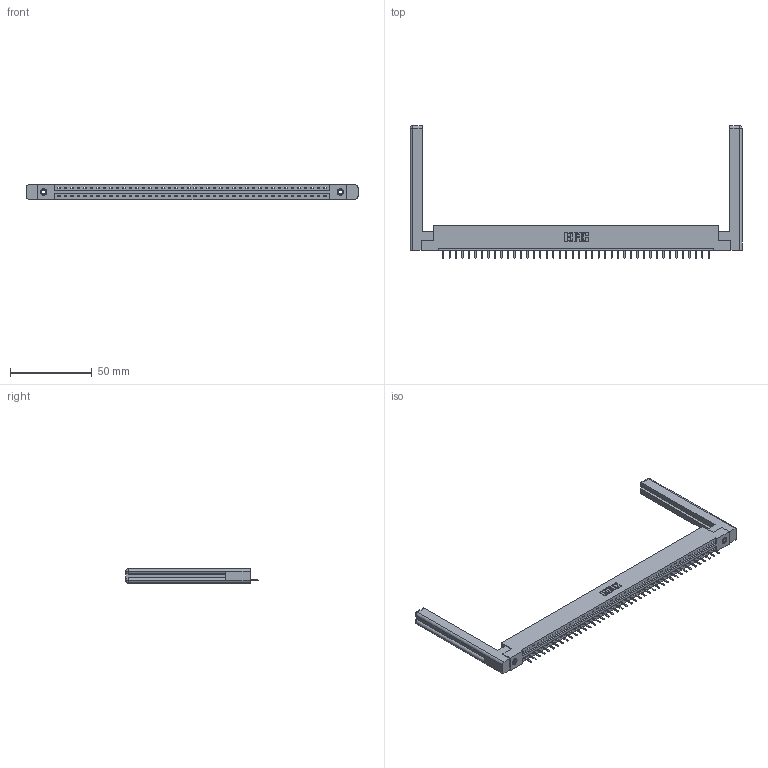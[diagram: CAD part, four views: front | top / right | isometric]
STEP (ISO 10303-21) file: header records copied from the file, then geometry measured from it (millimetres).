
FILE_DESCRIPTION (( 'STEP AP203' ), '1' );
FILE_NAME ('387-042-520-158.STEP', '2019-10-04T20:26:31', ( '' ), ( '' ), 'SwSTEP 2.0', 'SolidWorks 2016', '' );
FILE_SCHEMA (( 'CONFIG_CONTROL_DESIGN' ));
Length unit declared in the file: inch
Products named in the file (5): 345-292-001_345-293-120; 307-220-058; 345-250-001_345-250-001-102; 387-042-520-158; 337 Part_Flush Mounting Lugs - 0.156 Dia-TI
Assembly tree (47 placements, depth 2):
  387-042-520-158
    337 Part_Flush Mounting Lugs - 0.156 Dia-TI
    345-292-001_345-293-120  x42
    345-250-001_345-250-001-102  x2
    307-220-058  x2
Bounding box: 203.05 x 81.11 x 9.4 mm (x, y, z)
Volume: 28144.7 mm3; surface area: 26460.5 mm2
Topology: 47 solids, 47 shells, 3028 faces, 8897 edges, 5806 vertices
Faces by surface type: plane 2170, cylinder 834, cone 12, torus 12
Entity records: 33968 total; most frequent: CARTESIAN_POINT 5927, ORIENTED_EDGE 5832, DIRECTION 4996, EDGE_CURVE 2916, LINE 2736, VECTOR 2736, VERTEX_POINT 1934, AXIS2_PLACEMENT_3D 1130
